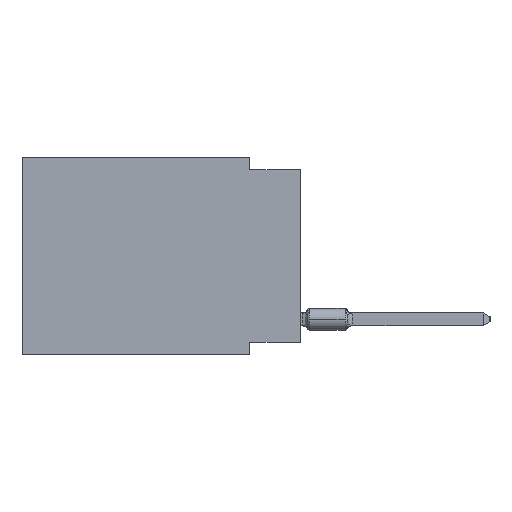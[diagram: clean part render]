
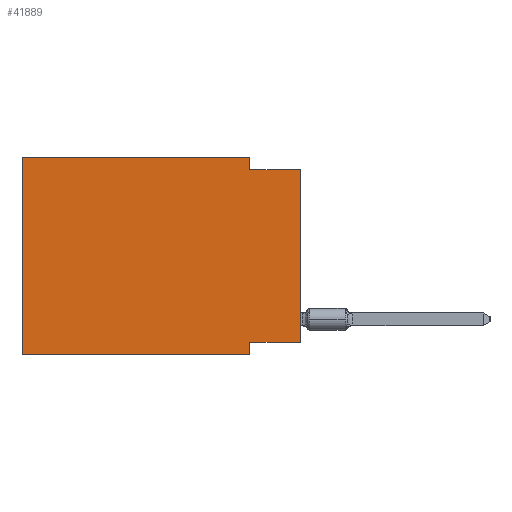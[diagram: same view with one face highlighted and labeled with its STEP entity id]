
A CAD part, left-side view. The second image highlights one B-rep face of the part: STEP entity #41889.
In plain terms, the highlighted planar face has unit normal (-1, 0, 0).
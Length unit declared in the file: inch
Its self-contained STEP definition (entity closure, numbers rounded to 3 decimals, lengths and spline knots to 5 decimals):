
#851 = CARTESIAN_POINT ( 'NONE',  ( 0., 0.1, -0.365 ) ) ;
#972 = CARTESIAN_POINT ( 'NONE',  ( 0., 0.55, 0. ) ) ;
#2021 = VECTOR ( 'NONE', #19722, 39.37008 ) ;
#2874 = ORIENTED_EDGE ( 'NONE', *, *, #55288, .F. ) ;
#3037 = ORIENTED_EDGE ( 'NONE', *, *, #18229, .T. ) ;
#4699 = VECTOR ( 'NONE', #5888, 39.37008 ) ;
#5011 = ORIENTED_EDGE ( 'NONE', *, *, #29394, .F. ) ;
#5888 = DIRECTION ( 'NONE',  ( 0., -1., 0. ) ) ;
#6031 = ORIENTED_EDGE ( 'NONE', *, *, #53994, .F. ) ;
#7586 = DIRECTION ( 'NONE',  ( 0., 0., -1. ) ) ;
#7662 = LINE ( 'NONE', #13567, #37965 ) ;
#8940 = VERTEX_POINT ( 'NONE', #24991 ) ;
#10198 = DIRECTION ( 'NONE',  ( 0., 0., 1. ) ) ;
#11185 = EDGE_CURVE ( 'NONE', #57044, #24860, #41508, .T. ) ;
#11286 = AXIS2_PLACEMENT_3D ( 'NONE', #28180, #12120, #7586 ) ;
#11523 = VECTOR ( 'NONE', #10198, 39.37008 ) ;
#12120 = DIRECTION ( 'NONE',  ( 1., 0., 0. ) ) ;
#12478 = FACE_OUTER_BOUND ( 'NONE', #34489, .T. ) ;
#13567 = CARTESIAN_POINT ( 'NONE',  ( 0., 0.55, -0.39 ) ) ;
#15352 = CARTESIAN_POINT ( 'NONE',  ( 0., 0., -0.025 ) ) ;
#15372 = CARTESIAN_POINT ( 'NONE',  ( 0., 0.1, -0.39 ) ) ;
#15696 = CARTESIAN_POINT ( 'NONE',  ( 0., 0., -0.365 ) ) ;
#15865 = CARTESIAN_POINT ( 'NONE',  ( 0., 0.55, 0. ) ) ;
#16437 = CARTESIAN_POINT ( 'NONE',  ( 0., 0., 0. ) ) ;
#17875 = ORIENTED_EDGE ( 'NONE', *, *, #26675, .F. ) ;
#18229 = EDGE_CURVE ( 'NONE', #30657, #52231, #7662, .T. ) ;
#18784 = DIRECTION ( 'NONE',  ( 0., -1., 0. ) ) ;
#19722 = DIRECTION ( 'NONE',  ( 0., 0., -1. ) ) ;
#20886 = LINE ( 'NONE', #58937, #58357 ) ;
#22597 = CARTESIAN_POINT ( 'NONE',  ( 0., 0., -0.365 ) ) ;
#23121 = ORIENTED_EDGE ( 'NONE', *, *, #11185, .F. ) ;
#24047 = VECTOR ( 'NONE', #41520, 39.37008 ) ;
#24573 = ORIENTED_EDGE ( 'NONE', *, *, #43000, .F. ) ;
#24860 = VERTEX_POINT ( 'NONE', #851 ) ;
#24991 = CARTESIAN_POINT ( 'NONE',  ( 0., 0.1, -0.025 ) ) ;
#26216 = EDGE_CURVE ( 'NONE', #57044, #41876, #68773, .T. ) ;
#26675 = EDGE_CURVE ( 'NONE', #24860, #52231, #20886, .T. ) ;
#28180 = CARTESIAN_POINT ( 'NONE',  ( 0., 0.55, 0. ) ) ;
#28514 = CARTESIAN_POINT ( 'NONE',  ( 0., 0., -0.025 ) ) ;
#29394 = EDGE_CURVE ( 'NONE', #8940, #41876, #52339, .T. ) ;
#30557 = CARTESIAN_POINT ( 'NONE',  ( 0., 0.1, 0. ) ) ;
#30657 = VERTEX_POINT ( 'NONE', #31886 ) ;
#31886 = CARTESIAN_POINT ( 'NONE',  ( 0., 0.55, -0.39 ) ) ;
#33098 = ORIENTED_EDGE ( 'NONE', *, *, #26216, .T. ) ;
#34200 = VECTOR ( 'NONE', #37945, 39.37008 ) ;
#34489 = EDGE_LOOP ( 'NONE', ( #33098, #5011, #2874, #24573, #6031, #3037, #17875, #23121 ) ) ;
#35055 = CARTESIAN_POINT ( 'NONE',  ( 0., 0.1, 0. ) ) ;
#36973 = DIRECTION ( 'NONE',  ( 0., 0., -1. ) ) ;
#37945 = DIRECTION ( 'NONE',  ( 0., 0., 1. ) ) ;
#37965 = VECTOR ( 'NONE', #18784, 39.37008 ) ;
#38971 = LINE ( 'NONE', #972, #34200 ) ;
#41508 = LINE ( 'NONE', #15696, #56388 ) ;
#41520 = DIRECTION ( 'NONE',  ( 0., -1., 0. ) ) ;
#41876 = VERTEX_POINT ( 'NONE', #28514 ) ;
#41889 = ADVANCED_FACE ( 'NONE', ( #12478 ), #60623, .F. ) ;
#42154 = CARTESIAN_POINT ( 'NONE',  ( 0., 0.55, 0. ) ) ;
#43000 = EDGE_CURVE ( 'NONE', #60930, #65843, #53671, .T. ) ;
#52231 = VERTEX_POINT ( 'NONE', #15372 ) ;
#52339 = LINE ( 'NONE', #15352, #24047 ) ;
#53671 = LINE ( 'NONE', #42154, #4699 ) ;
#53994 = EDGE_CURVE ( 'NONE', #30657, #60930, #38971, .T. ) ;
#55288 = EDGE_CURVE ( 'NONE', #65843, #8940, #61631, .T. ) ;
#56388 = VECTOR ( 'NONE', #62801, 39.37008 ) ;
#57044 = VERTEX_POINT ( 'NONE', #22597 ) ;
#58357 = VECTOR ( 'NONE', #36973, 39.37008 ) ;
#58937 = CARTESIAN_POINT ( 'NONE',  ( 0., 0.1, -0.39 ) ) ;
#60623 = PLANE ( 'NONE',  #11286 ) ;
#60930 = VERTEX_POINT ( 'NONE', #15865 ) ;
#61631 = LINE ( 'NONE', #30557, #2021 ) ;
#62801 = DIRECTION ( 'NONE',  ( 0., 1., 0. ) ) ;
#65843 = VERTEX_POINT ( 'NONE', #35055 ) ;
#68773 = LINE ( 'NONE', #16437, #11523 ) ;
